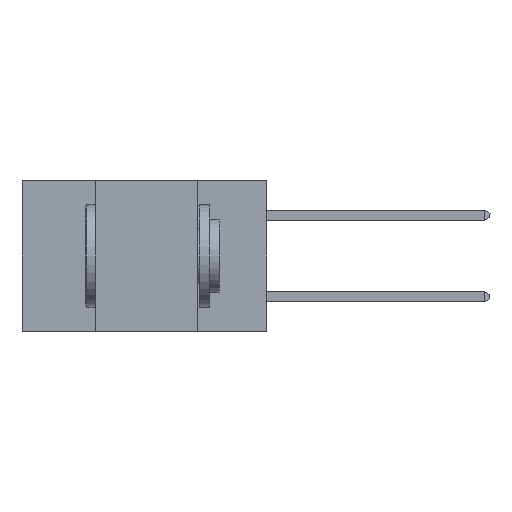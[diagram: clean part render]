
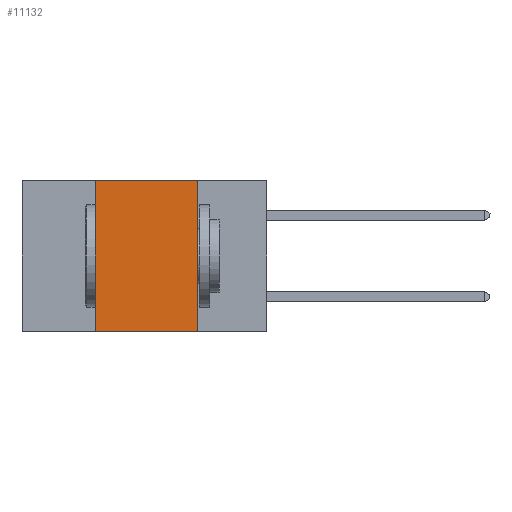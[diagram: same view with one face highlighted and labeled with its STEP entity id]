
A CAD part, left-side view. The second image highlights one B-rep face of the part: STEP entity #11132.
In plain terms, the highlighted planar face has unit normal (-1, 0, 0).
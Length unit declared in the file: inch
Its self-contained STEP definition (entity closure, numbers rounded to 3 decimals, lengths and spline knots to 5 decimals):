
#180 = VERTEX_POINT ( 'NONE', #9578 ) ;
#299 = EDGE_CURVE ( 'NONE', #180, #12088, #1500, .T. ) ;
#514 = VERTEX_POINT ( 'NONE', #6140 ) ;
#1312 = CARTESIAN_POINT ( 'NONE',  ( 0., 0.42, 0. ) ) ;
#1393 = DIRECTION ( 'NONE',  ( 0., 0., 1. ) ) ;
#1500 = LINE ( 'NONE', #10411, #10705 ) ;
#1722 = VERTEX_POINT ( 'NONE', #10078 ) ;
#2445 = AXIS2_PLACEMENT_3D ( 'NONE', #9809, #3271, #9842 ) ;
#2663 = EDGE_CURVE ( 'NONE', #514, #1722, #4399, .T. ) ;
#3271 = DIRECTION ( 'NONE',  ( 1., 0., 0. ) ) ;
#3536 = EDGE_CURVE ( 'NONE', #514, #12088, #6640, .T. ) ;
#4241 = CARTESIAN_POINT ( 'NONE',  ( 0., 0.17, -0.37 ) ) ;
#4399 = LINE ( 'NONE', #1312, #4705 ) ;
#4566 = ORIENTED_EDGE ( 'NONE', *, *, #7241, .F. ) ;
#4585 = VECTOR ( 'NONE', #8116, 39.37008 ) ;
#4705 = VECTOR ( 'NONE', #1393, 39.37008 ) ;
#4821 = DIRECTION ( 'NONE',  ( 0., 0., -1. ) ) ;
#5040 = FACE_OUTER_BOUND ( 'NONE', #6094, .T. ) ;
#5398 = DIRECTION ( 'NONE',  ( 0., -1., 0. ) ) ;
#5566 = CARTESIAN_POINT ( 'NONE',  ( 0., 0.6, -0.37 ) ) ;
#6094 = EDGE_LOOP ( 'NONE', ( #9222, #4566, #7109, #9505 ) ) ;
#6140 = CARTESIAN_POINT ( 'NONE',  ( 0., 0.42, -0.37 ) ) ;
#6640 = LINE ( 'NONE', #5566, #11137 ) ;
#7109 = ORIENTED_EDGE ( 'NONE', *, *, #2663, .F. ) ;
#7241 = EDGE_CURVE ( 'NONE', #1722, #180, #9518, .T. ) ;
#8116 = DIRECTION ( 'NONE',  ( 0., -1., 0. ) ) ;
#8919 = PLANE ( 'NONE',  #2445 ) ;
#8967 = CARTESIAN_POINT ( 'NONE',  ( 0., 0.6, 0. ) ) ;
#9222 = ORIENTED_EDGE ( 'NONE', *, *, #299, .F. ) ;
#9505 = ORIENTED_EDGE ( 'NONE', *, *, #3536, .T. ) ;
#9518 = LINE ( 'NONE', #8967, #4585 ) ;
#9578 = CARTESIAN_POINT ( 'NONE',  ( 0., 0.17, 0. ) ) ;
#9809 = CARTESIAN_POINT ( 'NONE',  ( 0., 0.6, 0. ) ) ;
#9842 = DIRECTION ( 'NONE',  ( 0., 0., -1. ) ) ;
#10078 = CARTESIAN_POINT ( 'NONE',  ( 0., 0.42, 0. ) ) ;
#10411 = CARTESIAN_POINT ( 'NONE',  ( 0., 0.17, 0. ) ) ;
#10705 = VECTOR ( 'NONE', #4821, 39.37008 ) ;
#11132 = ADVANCED_FACE ( 'NONE', ( #5040 ), #8919, .F. ) ;
#11137 = VECTOR ( 'NONE', #5398, 39.37008 ) ;
#12088 = VERTEX_POINT ( 'NONE', #4241 ) ;
